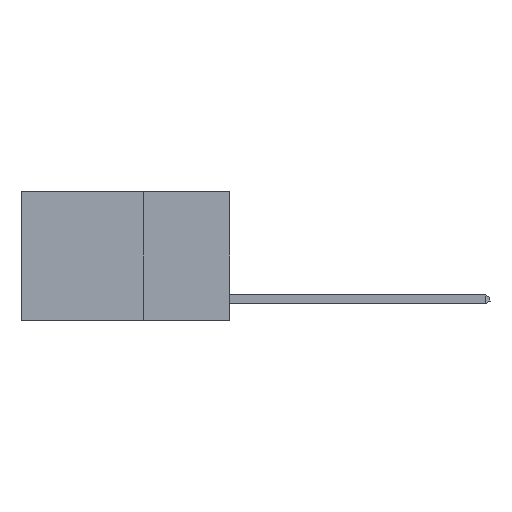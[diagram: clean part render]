
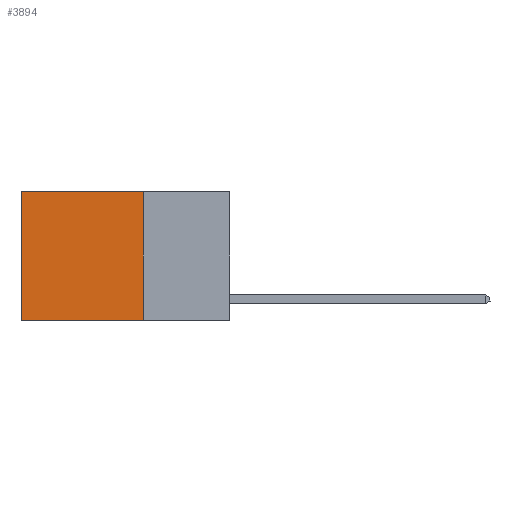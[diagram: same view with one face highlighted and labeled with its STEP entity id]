
A CAD part, left-side view. The second image highlights one B-rep face of the part: STEP entity #3894.
In plain terms, the highlighted planar face has unit normal (-1, 0, 0).
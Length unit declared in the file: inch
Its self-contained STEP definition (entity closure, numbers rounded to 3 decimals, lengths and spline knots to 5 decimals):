
#205 = ORIENTED_EDGE ( 'NONE', *, *, #10870, .F. ) ;
#1053 = VERTEX_POINT ( 'NONE', #11120 ) ;
#1109 = EDGE_LOOP ( 'NONE', ( #3315, #16081, #205, #12714 ) ) ;
#2546 = LINE ( 'NONE', #15283, #4007 ) ;
#3315 = ORIENTED_EDGE ( 'NONE', *, *, #12853, .T. ) ;
#3894 = ADVANCED_FACE ( 'NONE', ( #14530 ), #7218, .F. ) ;
#4007 = VECTOR ( 'NONE', #11086, 39.37008 ) ;
#4203 = DIRECTION ( 'NONE',  ( 1., 0., 0. ) ) ;
#6217 = EDGE_CURVE ( 'NONE', #1053, #10418, #11885, .T. ) ;
#6663 = LINE ( 'NONE', #12280, #9661 ) ;
#6748 = EDGE_CURVE ( 'NONE', #8379, #11684, #16713, .T. ) ;
#7218 = PLANE ( 'NONE',  #17959 ) ;
#7668 = DIRECTION ( 'NONE',  ( 0., 1., 0. ) ) ;
#7912 = DIRECTION ( 'NONE',  ( 0., 1., 0. ) ) ;
#8064 = DIRECTION ( 'NONE',  ( 0., 0., -1. ) ) ;
#8379 = VERTEX_POINT ( 'NONE', #14643 ) ;
#9586 = VECTOR ( 'NONE', #7668, 39.37008 ) ;
#9661 = VECTOR ( 'NONE', #8064, 39.37008 ) ;
#10418 = VERTEX_POINT ( 'NONE', #13979 ) ;
#10870 = EDGE_CURVE ( 'NONE', #8379, #1053, #6663, .T. ) ;
#11086 = DIRECTION ( 'NONE',  ( 0., 0., -1. ) ) ;
#11120 = CARTESIAN_POINT ( 'NONE',  ( 0.2625, 0.25, -0.37 ) ) ;
#11256 = DIRECTION ( 'NONE',  ( 0., 0., -1. ) ) ;
#11684 = VERTEX_POINT ( 'NONE', #16815 ) ;
#11885 = LINE ( 'NONE', #16449, #9586 ) ;
#12280 = CARTESIAN_POINT ( 'NONE',  ( 0.2625, 0.25, 0. ) ) ;
#12575 = CARTESIAN_POINT ( 'NONE',  ( 0.2625, 0.25, 0. ) ) ;
#12650 = CARTESIAN_POINT ( 'NONE',  ( 0.2625, 0.25, 0. ) ) ;
#12714 = ORIENTED_EDGE ( 'NONE', *, *, #6748, .T. ) ;
#12853 = EDGE_CURVE ( 'NONE', #11684, #10418, #2546, .T. ) ;
#13979 = CARTESIAN_POINT ( 'NONE',  ( 0.2625, 0.6, -0.37 ) ) ;
#14530 = FACE_OUTER_BOUND ( 'NONE', #1109, .T. ) ;
#14643 = CARTESIAN_POINT ( 'NONE',  ( 0.2625, 0.25, 0. ) ) ;
#14964 = VECTOR ( 'NONE', #7912, 39.37008 ) ;
#15283 = CARTESIAN_POINT ( 'NONE',  ( 0.2625, 0.6, 0. ) ) ;
#16081 = ORIENTED_EDGE ( 'NONE', *, *, #6217, .F. ) ;
#16449 = CARTESIAN_POINT ( 'NONE',  ( 0.2625, 0.25, -0.37 ) ) ;
#16713 = LINE ( 'NONE', #12575, #14964 ) ;
#16815 = CARTESIAN_POINT ( 'NONE',  ( 0.2625, 0.6, 0. ) ) ;
#17959 = AXIS2_PLACEMENT_3D ( 'NONE', #12650, #4203, #11256 ) ;
